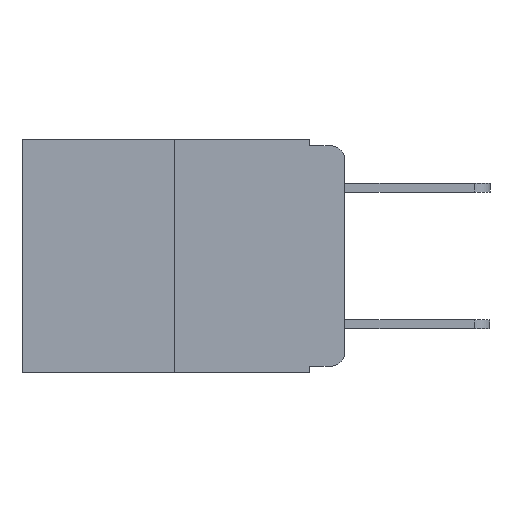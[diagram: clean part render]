
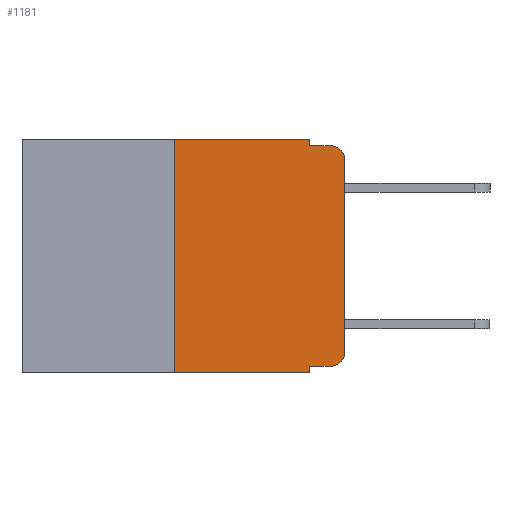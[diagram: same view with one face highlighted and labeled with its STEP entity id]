
A CAD part, left-side view. The second image highlights one B-rep face of the part: STEP entity #1181.
In plain terms, the highlighted planar face has unit normal (-1, 0, 0).
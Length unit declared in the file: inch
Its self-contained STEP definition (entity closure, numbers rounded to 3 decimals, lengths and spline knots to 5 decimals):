
#203 = DIRECTION ( 'NONE',  ( 0., 0., -1. ) ) ;
#556 = DIRECTION ( 'NONE',  ( -1., 0., 0. ) ) ;
#1047 = EDGE_CURVE ( 'NONE', #10806, #6051, #21319, .T. ) ;
#1170 = CIRCLE ( 'NONE', #12157, 0.02 ) ;
#1181 = ADVANCED_FACE ( 'NONE', ( #23490 ), #12176, .F. ) ;
#1286 = LINE ( 'NONE', #6481, #15377 ) ;
#1479 = CARTESIAN_POINT ( 'NONE',  ( 0., 0.473, 0. ) ) ;
#1685 = DIRECTION ( 'NONE',  ( 0., -1., 0. ) ) ;
#3963 = CARTESIAN_POINT ( 'NONE',  ( 0., 0.25, 0. ) ) ;
#4734 = VECTOR ( 'NONE', #10032, 39.37008 ) ;
#4992 = EDGE_LOOP ( 'NONE', ( #19304, #25139, #8396, #24870, #24571, #9956, #5996, #13554, #10834, #12920 ) ) ;
#5096 = VECTOR ( 'NONE', #13387, 39.37008 ) ;
#5456 = VECTOR ( 'NONE', #13474, 39.37008 ) ;
#5996 = ORIENTED_EDGE ( 'NONE', *, *, #19434, .T. ) ;
#6051 = VERTEX_POINT ( 'NONE', #15481 ) ;
#6481 = CARTESIAN_POINT ( 'NONE',  ( 0., 0.051, 0. ) ) ;
#6531 = VERTEX_POINT ( 'NONE', #18918 ) ;
#7173 = CARTESIAN_POINT ( 'NONE',  ( 0., 0.25, 0. ) ) ;
#7547 = VERTEX_POINT ( 'NONE', #19855 ) ;
#8009 = DIRECTION ( 'NONE',  ( 0., 0., -1. ) ) ;
#8045 = CIRCLE ( 'NONE', #16481, 0.02 ) ;
#8254 = EDGE_CURVE ( 'NONE', #20555, #13952, #15702, .T. ) ;
#8349 = CARTESIAN_POINT ( 'NONE',  ( 0., 0.02, -0.03 ) ) ;
#8396 = ORIENTED_EDGE ( 'NONE', *, *, #24177, .F. ) ;
#8490 = DIRECTION ( 'NONE',  ( 0., 0., -1. ) ) ;
#8517 = EDGE_CURVE ( 'NONE', #21060, #7547, #1286, .T. ) ;
#9956 = ORIENTED_EDGE ( 'NONE', *, *, #21680, .F. ) ;
#10032 = DIRECTION ( 'NONE',  ( 0., 0., 1. ) ) ;
#10159 = LINE ( 'NONE', #21001, #19483 ) ;
#10377 = DIRECTION ( 'NONE',  ( 0., 0., -1. ) ) ;
#10452 = CARTESIAN_POINT ( 'NONE',  ( 0., 0.051, -0.333 ) ) ;
#10566 = EDGE_CURVE ( 'NONE', #11554, #20555, #1170, .T. ) ;
#10806 = VERTEX_POINT ( 'NONE', #7173 ) ;
#10834 = ORIENTED_EDGE ( 'NONE', *, *, #23396, .T. ) ;
#10904 = VECTOR ( 'NONE', #21546, 39.37008 ) ;
#11233 = EDGE_CURVE ( 'NONE', #13952, #6531, #8045, .T. ) ;
#11530 = LINE ( 'NONE', #19577, #10904 ) ;
#11554 = VERTEX_POINT ( 'NONE', #25158 ) ;
#12157 = AXIS2_PLACEMENT_3D ( 'NONE', #12594, #556, #14596 ) ;
#12176 = PLANE ( 'NONE',  #23132 ) ;
#12255 = DIRECTION ( 'NONE',  ( 1., 0., 0. ) ) ;
#12594 = CARTESIAN_POINT ( 'NONE',  ( 0., 0.02, -0.313 ) ) ;
#12920 = ORIENTED_EDGE ( 'NONE', *, *, #10566, .T. ) ;
#13276 = CARTESIAN_POINT ( 'NONE',  ( 0., 0.25, -0.343 ) ) ;
#13387 = DIRECTION ( 'NONE',  ( 0., 0., 1. ) ) ;
#13474 = DIRECTION ( 'NONE',  ( 0., -1., 0. ) ) ;
#13554 = ORIENTED_EDGE ( 'NONE', *, *, #8517, .F. ) ;
#13724 = LINE ( 'NONE', #23572, #18373 ) ;
#13839 = VECTOR ( 'NONE', #8009, 39.37008 ) ;
#13952 = VERTEX_POINT ( 'NONE', #24171 ) ;
#14596 = DIRECTION ( 'NONE',  ( 0., 0., -1. ) ) ;
#15377 = VECTOR ( 'NONE', #8490, 39.37008 ) ;
#15387 = CARTESIAN_POINT ( 'NONE',  ( 0., 0., 0. ) ) ;
#15481 = CARTESIAN_POINT ( 'NONE',  ( 0., 0.051, 0. ) ) ;
#15702 = LINE ( 'NONE', #15387, #5096 ) ;
#16159 = CARTESIAN_POINT ( 'NONE',  ( 0., 0.473, 0. ) ) ;
#16481 = AXIS2_PLACEMENT_3D ( 'NONE', #8349, #22241, #10377 ) ;
#16827 = CARTESIAN_POINT ( 'NONE',  ( 0., 0.051, -0.01 ) ) ;
#17930 = CARTESIAN_POINT ( 'NONE',  ( 0., 0.051, 0. ) ) ;
#18373 = VECTOR ( 'NONE', #1685, 39.37008 ) ;
#18918 = CARTESIAN_POINT ( 'NONE',  ( 0., 0.02, -0.01 ) ) ;
#19304 = ORIENTED_EDGE ( 'NONE', *, *, #8254, .T. ) ;
#19434 = EDGE_CURVE ( 'NONE', #20121, #7547, #10159, .T. ) ;
#19483 = VECTOR ( 'NONE', #23001, 39.37008 ) ;
#19577 = CARTESIAN_POINT ( 'NONE',  ( 0., 0.051, -0.01 ) ) ;
#19855 = CARTESIAN_POINT ( 'NONE',  ( 0., 0.051, -0.343 ) ) ;
#20121 = VERTEX_POINT ( 'NONE', #13276 ) ;
#20361 = EDGE_CURVE ( 'NONE', #6051, #25114, #24359, .T. ) ;
#20555 = VERTEX_POINT ( 'NONE', #22502 ) ;
#20616 = LINE ( 'NONE', #3963, #4734 ) ;
#21001 = CARTESIAN_POINT ( 'NONE',  ( 0., 0.473, -0.343 ) ) ;
#21060 = VERTEX_POINT ( 'NONE', #10452 ) ;
#21319 = LINE ( 'NONE', #1479, #5456 ) ;
#21546 = DIRECTION ( 'NONE',  ( 0., -1., 0. ) ) ;
#21680 = EDGE_CURVE ( 'NONE', #20121, #10806, #20616, .T. ) ;
#22241 = DIRECTION ( 'NONE',  ( -1., 0., 0. ) ) ;
#22502 = CARTESIAN_POINT ( 'NONE',  ( 0., 0., -0.313 ) ) ;
#23001 = DIRECTION ( 'NONE',  ( 0., -1., 0. ) ) ;
#23132 = AXIS2_PLACEMENT_3D ( 'NONE', #16159, #12255, #203 ) ;
#23396 = EDGE_CURVE ( 'NONE', #21060, #11554, #13724, .T. ) ;
#23490 = FACE_OUTER_BOUND ( 'NONE', #4992, .T. ) ;
#23572 = CARTESIAN_POINT ( 'NONE',  ( 0., 0.051, -0.333 ) ) ;
#24171 = CARTESIAN_POINT ( 'NONE',  ( 0., 0., -0.03 ) ) ;
#24177 = EDGE_CURVE ( 'NONE', #25114, #6531, #11530, .T. ) ;
#24359 = LINE ( 'NONE', #17930, #13839 ) ;
#24571 = ORIENTED_EDGE ( 'NONE', *, *, #1047, .F. ) ;
#24870 = ORIENTED_EDGE ( 'NONE', *, *, #20361, .F. ) ;
#25114 = VERTEX_POINT ( 'NONE', #16827 ) ;
#25139 = ORIENTED_EDGE ( 'NONE', *, *, #11233, .T. ) ;
#25158 = CARTESIAN_POINT ( 'NONE',  ( 0., 0.02, -0.333 ) ) ;
